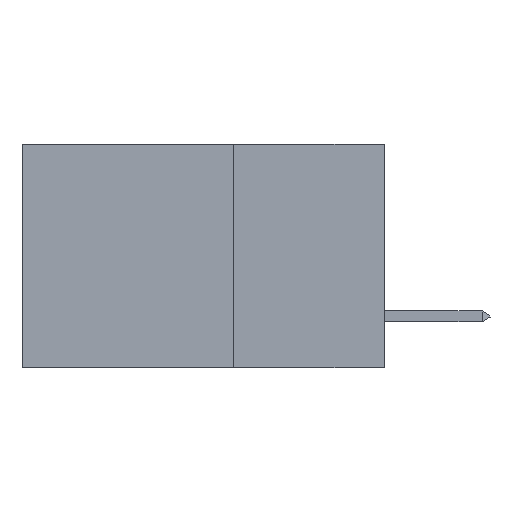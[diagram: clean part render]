
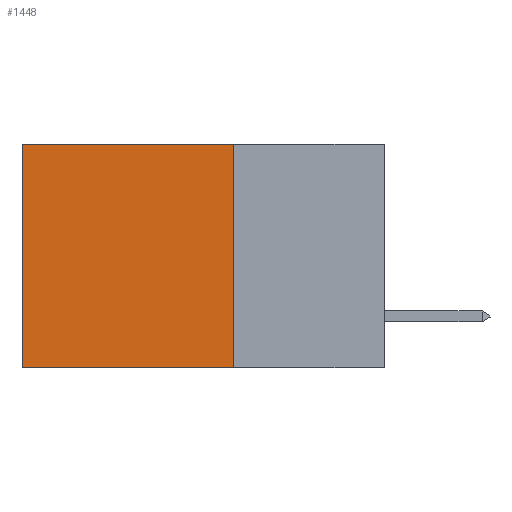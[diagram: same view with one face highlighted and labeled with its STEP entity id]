
A CAD part, left-side view. The second image highlights one B-rep face of the part: STEP entity #1448.
In plain terms, the highlighted planar face has unit normal (-1, 0, 0).
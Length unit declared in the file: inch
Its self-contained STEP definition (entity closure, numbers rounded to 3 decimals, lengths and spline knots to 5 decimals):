
#46 = DIRECTION ( 'NONE',  ( 0., 0., -1. ) ) ;
#296 = CARTESIAN_POINT ( 'NONE',  ( 0.2875, 0.25, 0. ) ) ;
#329 = VECTOR ( 'NONE', #6117, 39.37008 ) ;
#704 = EDGE_CURVE ( 'NONE', #15986, #12321, #796, .T. ) ;
#796 = LINE ( 'NONE', #17835, #329 ) ;
#871 = EDGE_CURVE ( 'NONE', #4115, #15986, #18781, .T. ) ;
#1448 = ADVANCED_FACE ( 'NONE', ( #17338 ), #7205, .F. ) ;
#1572 = CARTESIAN_POINT ( 'NONE',  ( 0.2875, 0.25, -0.37 ) ) ;
#2519 = LINE ( 'NONE', #15062, #16546 ) ;
#2764 = ORIENTED_EDGE ( 'NONE', *, *, #4258, .T. ) ;
#2980 = LINE ( 'NONE', #11437, #14403 ) ;
#4115 = VERTEX_POINT ( 'NONE', #16121 ) ;
#4258 = EDGE_CURVE ( 'NONE', #16641, #12321, #2519, .T. ) ;
#5090 = ORIENTED_EDGE ( 'NONE', *, *, #6208, .T. ) ;
#5509 = CARTESIAN_POINT ( 'NONE',  ( 0.2875, 0.25, 0. ) ) ;
#6117 = DIRECTION ( 'NONE',  ( 0., 1., 0. ) ) ;
#6208 = EDGE_CURVE ( 'NONE', #4115, #16641, #2980, .T. ) ;
#7011 = DIRECTION ( 'NONE',  ( 0., 1., 0. ) ) ;
#7205 = PLANE ( 'NONE',  #14272 ) ;
#7755 = CARTESIAN_POINT ( 'NONE',  ( 0.2875, 0.6, 0. ) ) ;
#9774 = ORIENTED_EDGE ( 'NONE', *, *, #871, .F. ) ;
#9916 = DIRECTION ( 'NONE',  ( 1., 0., 0. ) ) ;
#11437 = CARTESIAN_POINT ( 'NONE',  ( 0.2875, 0.25, 0. ) ) ;
#12321 = VERTEX_POINT ( 'NONE', #12399 ) ;
#12399 = CARTESIAN_POINT ( 'NONE',  ( 0.2875, 0.6, -0.37 ) ) ;
#14272 = AXIS2_PLACEMENT_3D ( 'NONE', #5509, #9916, #14350 ) ;
#14350 = DIRECTION ( 'NONE',  ( 0., 0., -1. ) ) ;
#14403 = VECTOR ( 'NONE', #7011, 39.37008 ) ;
#14563 = VECTOR ( 'NONE', #18248, 39.37008 ) ;
#15062 = CARTESIAN_POINT ( 'NONE',  ( 0.2875, 0.6, 0. ) ) ;
#15984 = EDGE_LOOP ( 'NONE', ( #2764, #17467, #9774, #5090 ) ) ;
#15986 = VERTEX_POINT ( 'NONE', #1572 ) ;
#16121 = CARTESIAN_POINT ( 'NONE',  ( 0.2875, 0.25, 0. ) ) ;
#16546 = VECTOR ( 'NONE', #46, 39.37008 ) ;
#16641 = VERTEX_POINT ( 'NONE', #7755 ) ;
#17338 = FACE_OUTER_BOUND ( 'NONE', #15984, .T. ) ;
#17467 = ORIENTED_EDGE ( 'NONE', *, *, #704, .F. ) ;
#17835 = CARTESIAN_POINT ( 'NONE',  ( 0.2875, 0.25, -0.37 ) ) ;
#18248 = DIRECTION ( 'NONE',  ( 0., 0., -1. ) ) ;
#18781 = LINE ( 'NONE', #296, #14563 ) ;
